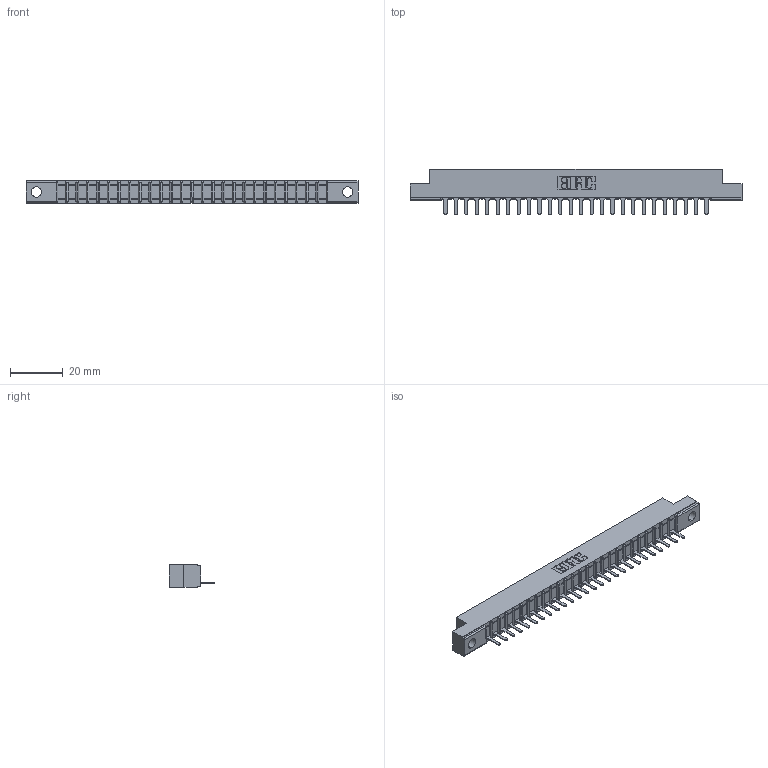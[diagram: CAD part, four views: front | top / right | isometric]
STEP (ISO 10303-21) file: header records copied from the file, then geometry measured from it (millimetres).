
FILE_DESCRIPTION (( 'STEP AP203' ), '1' );
FILE_NAME ('357-026-425-104.STEP', '2020-10-01T16:16:46', ( '' ), ( '' ), 'SwSTEP 2.0', 'SolidWorks 2020', '' );
FILE_SCHEMA (( 'CONFIG_CONTROL_DESIGN' ));
Length unit declared in the file: inch
Products named in the file (3): 307-290-001_525; 307 Part_.156 Dia Mounting Holes; 357-026-425-104
Assembly tree (27 placements, depth 2):
  357-026-425-104
    307 Part_.156 Dia Mounting Holes
    307-290-001_525  x26
Bounding box: 126.03 x 17.42 x 8.71 mm (x, y, z)
Volume: 7821.2 mm3; surface area: 12002.4 mm2
Topology: 27 solids, 27 shells, 1615 faces, 4571 edges, 2938 vertices
Faces by surface type: plane 1046, cylinder 515, sphere 54
Entity records: 24648 total; most frequent: CARTESIAN_POINT 4150, ORIENTED_EDGE 4134, DIRECTION 4037, EDGE_CURVE 2067, LINE 1587, VECTOR 1587, VERTEX_POINT 1338, AXIS2_PLACEMENT_3D 1225
